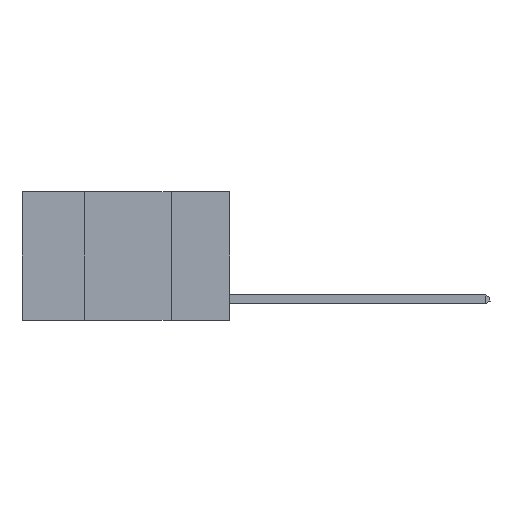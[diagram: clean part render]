
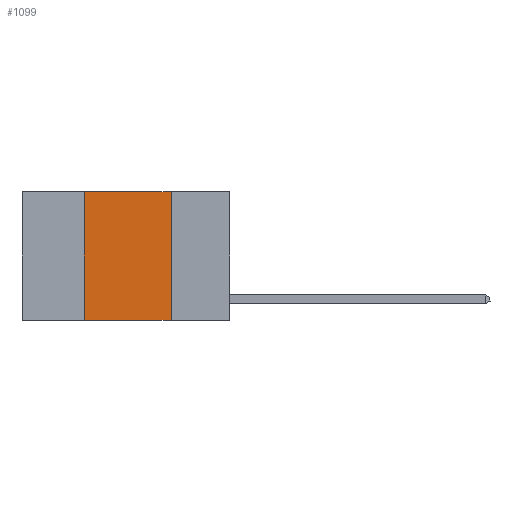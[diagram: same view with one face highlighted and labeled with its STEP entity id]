
A CAD part, left-side view. The second image highlights one B-rep face of the part: STEP entity #1099.
In plain terms, the highlighted planar face has unit normal (-1, 0, 0).
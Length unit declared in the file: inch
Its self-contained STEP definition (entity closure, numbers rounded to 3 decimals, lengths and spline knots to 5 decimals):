
#28 = DIRECTION ( 'NONE',  ( 0., -1., 0. ) ) ;
#95 = CARTESIAN_POINT ( 'NONE',  ( 0., 0.42, 0. ) ) ;
#362 = ORIENTED_EDGE ( 'NONE', *, *, #4926, .F. ) ;
#1099 = ADVANCED_FACE ( 'NONE', ( #7786 ), #14771, .F. ) ;
#1149 = ORIENTED_EDGE ( 'NONE', *, *, #11177, .T. ) ;
#2299 = CARTESIAN_POINT ( 'NONE',  ( 0., 0.42, 0. ) ) ;
#3176 = VERTEX_POINT ( 'NONE', #5543 ) ;
#3621 = CARTESIAN_POINT ( 'NONE',  ( 0., 0.6, 0. ) ) ;
#3795 = LINE ( 'NONE', #10864, #17271 ) ;
#3954 = EDGE_CURVE ( 'NONE', #15870, #11543, #11539, .T. ) ;
#4282 = CARTESIAN_POINT ( 'NONE',  ( 0., 0.17, -0.37 ) ) ;
#4437 = ORIENTED_EDGE ( 'NONE', *, *, #6279, .F. ) ;
#4926 = EDGE_CURVE ( 'NONE', #11543, #3176, #17074, .T. ) ;
#5057 = DIRECTION ( 'NONE',  ( 0., -1., 0. ) ) ;
#5200 = AXIS2_PLACEMENT_3D ( 'NONE', #3621, #6552, #16150 ) ;
#5543 = CARTESIAN_POINT ( 'NONE',  ( 0., 0.17, 0. ) ) ;
#6117 = VECTOR ( 'NONE', #5057, 39.37008 ) ;
#6279 = EDGE_CURVE ( 'NONE', #3176, #11768, #3795, .T. ) ;
#6552 = DIRECTION ( 'NONE',  ( 1., 0., 0. ) ) ;
#7254 = CARTESIAN_POINT ( 'NONE',  ( 0., 0.6, -0.37 ) ) ;
#7458 = VECTOR ( 'NONE', #11420, 39.37008 ) ;
#7786 = FACE_OUTER_BOUND ( 'NONE', #12219, .T. ) ;
#10864 = CARTESIAN_POINT ( 'NONE',  ( 0., 0.17, 0. ) ) ;
#11177 = EDGE_CURVE ( 'NONE', #15870, #11768, #14238, .T. ) ;
#11420 = DIRECTION ( 'NONE',  ( 0., 0., 1. ) ) ;
#11539 = LINE ( 'NONE', #95, #7458 ) ;
#11543 = VERTEX_POINT ( 'NONE', #2299 ) ;
#11768 = VERTEX_POINT ( 'NONE', #4282 ) ;
#12068 = CARTESIAN_POINT ( 'NONE',  ( 0., 0.6, 0. ) ) ;
#12219 = EDGE_LOOP ( 'NONE', ( #4437, #362, #16767, #1149 ) ) ;
#12259 = DIRECTION ( 'NONE',  ( 0., 0., -1. ) ) ;
#13398 = VECTOR ( 'NONE', #28, 39.37008 ) ;
#14238 = LINE ( 'NONE', #7254, #13398 ) ;
#14771 = PLANE ( 'NONE',  #5200 ) ;
#15870 = VERTEX_POINT ( 'NONE', #17174 ) ;
#16150 = DIRECTION ( 'NONE',  ( 0., 0., -1. ) ) ;
#16767 = ORIENTED_EDGE ( 'NONE', *, *, #3954, .F. ) ;
#17074 = LINE ( 'NONE', #12068, #6117 ) ;
#17174 = CARTESIAN_POINT ( 'NONE',  ( 0., 0.42, -0.37 ) ) ;
#17271 = VECTOR ( 'NONE', #12259, 39.37008 ) ;
